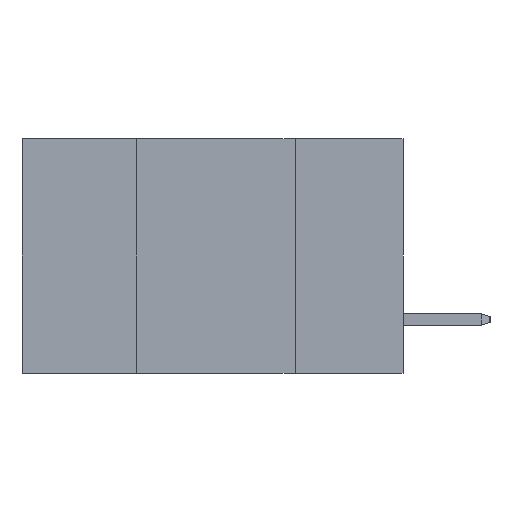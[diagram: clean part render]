
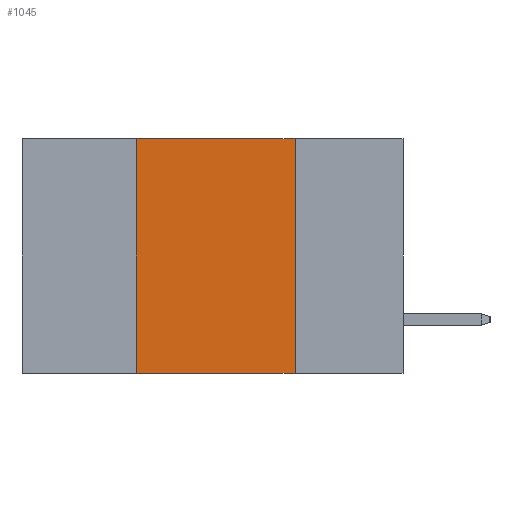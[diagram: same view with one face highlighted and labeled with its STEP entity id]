
A CAD part, left-side view. The second image highlights one B-rep face of the part: STEP entity #1045.
In plain terms, the highlighted planar face has unit normal (-1, 0, 0).
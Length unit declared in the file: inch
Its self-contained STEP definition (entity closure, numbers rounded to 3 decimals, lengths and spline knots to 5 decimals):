
#252 = CARTESIAN_POINT ( 'NONE',  ( 0., 0.6, 0. ) ) ;
#261 = VECTOR ( 'NONE', #12789, 39.37008 ) ;
#386 = ORIENTED_EDGE ( 'NONE', *, *, #11561, .F. ) ;
#693 = CARTESIAN_POINT ( 'NONE',  ( 0., 0.6, -0.37 ) ) ;
#1045 = ADVANCED_FACE ( 'NONE', ( #7204 ), #10456, .F. ) ;
#1491 = CARTESIAN_POINT ( 'NONE',  ( 0., 0.6, 0. ) ) ;
#1538 = VERTEX_POINT ( 'NONE', #4277 ) ;
#1580 = ORIENTED_EDGE ( 'NONE', *, *, #7252, .T. ) ;
#1592 = VECTOR ( 'NONE', #2624, 39.37008 ) ;
#2564 = LINE ( 'NONE', #8811, #1592 ) ;
#2604 = CARTESIAN_POINT ( 'NONE',  ( 0., 0.17, -0.37 ) ) ;
#2624 = DIRECTION ( 'NONE',  ( 0., 0., -1. ) ) ;
#3126 = CARTESIAN_POINT ( 'NONE',  ( 0., 0.42, 0. ) ) ;
#3196 = DIRECTION ( 'NONE',  ( 0., 0., 1. ) ) ;
#3267 = VERTEX_POINT ( 'NONE', #9204 ) ;
#4277 = CARTESIAN_POINT ( 'NONE',  ( 0., 0.17, 0. ) ) ;
#4389 = EDGE_CURVE ( 'NONE', #3267, #1538, #10693, .T. ) ;
#4734 = CARTESIAN_POINT ( 'NONE',  ( 0., 0.42, -0.37 ) ) ;
#4763 = DIRECTION ( 'NONE',  ( 0., -1., 0. ) ) ;
#5091 = ORIENTED_EDGE ( 'NONE', *, *, #4389, .F. ) ;
#5649 = LINE ( 'NONE', #693, #8214 ) ;
#5864 = VERTEX_POINT ( 'NONE', #2604 ) ;
#7204 = FACE_OUTER_BOUND ( 'NONE', #10685, .T. ) ;
#7252 = EDGE_CURVE ( 'NONE', #7761, #5864, #5649, .T. ) ;
#7761 = VERTEX_POINT ( 'NONE', #4734 ) ;
#8214 = VECTOR ( 'NONE', #4763, 39.37008 ) ;
#8691 = ORIENTED_EDGE ( 'NONE', *, *, #8782, .F. ) ;
#8782 = EDGE_CURVE ( 'NONE', #1538, #5864, #2564, .T. ) ;
#8811 = CARTESIAN_POINT ( 'NONE',  ( 0., 0.17, 0. ) ) ;
#8926 = VECTOR ( 'NONE', #3196, 39.37008 ) ;
#9204 = CARTESIAN_POINT ( 'NONE',  ( 0., 0.42, 0. ) ) ;
#9232 = LINE ( 'NONE', #3126, #8926 ) ;
#10456 = PLANE ( 'NONE',  #12170 ) ;
#10685 = EDGE_LOOP ( 'NONE', ( #8691, #5091, #386, #1580 ) ) ;
#10693 = LINE ( 'NONE', #1491, #261 ) ;
#11539 = DIRECTION ( 'NONE',  ( 1., 0., 0. ) ) ;
#11561 = EDGE_CURVE ( 'NONE', #7761, #3267, #9232, .T. ) ;
#11595 = DIRECTION ( 'NONE',  ( 0., 0., -1. ) ) ;
#12170 = AXIS2_PLACEMENT_3D ( 'NONE', #252, #11539, #11595 ) ;
#12789 = DIRECTION ( 'NONE',  ( 0., -1., 0. ) ) ;
